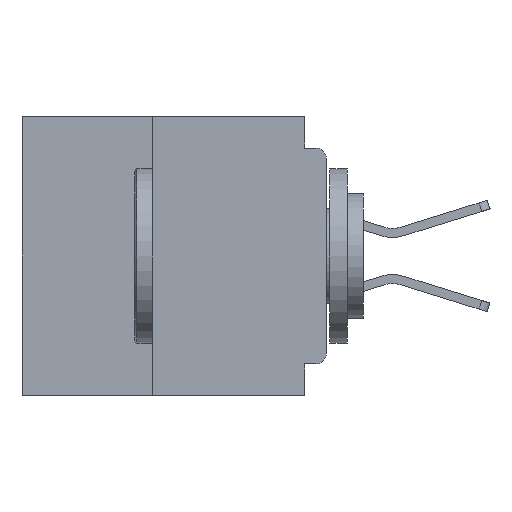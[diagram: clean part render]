
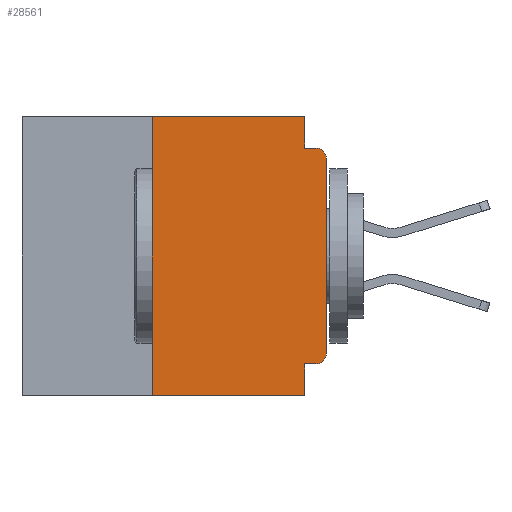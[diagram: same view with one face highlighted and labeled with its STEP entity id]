
A CAD part, left-side view. The second image highlights one B-rep face of the part: STEP entity #28561.
In plain terms, the highlighted planar face has unit normal (-1, 0, 0).
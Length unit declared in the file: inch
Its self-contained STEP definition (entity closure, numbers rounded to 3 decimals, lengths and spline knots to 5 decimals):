
#511 = ORIENTED_EDGE ( 'NONE', *, *, #9214, .T. ) ;
#1726 = VERTEX_POINT ( 'NONE', #33246 ) ;
#2229 = CARTESIAN_POINT ( 'NONE',  ( 0., 0.015, -0.34 ) ) ;
#2244 = DIRECTION ( 'NONE',  ( 0., 0., -1. ) ) ;
#4457 = VERTEX_POINT ( 'NONE', #42054 ) ;
#4629 = LINE ( 'NONE', #41701, #37160 ) ;
#4651 = CIRCLE ( 'NONE', #56440, 0.015 ) ;
#6211 = ORIENTED_EDGE ( 'NONE', *, *, #53278, .T. ) ;
#6963 = DIRECTION ( 'NONE',  ( 0., 0., -1. ) ) ;
#7548 = VERTEX_POINT ( 'NONE', #15556 ) ;
#9214 = EDGE_CURVE ( 'NONE', #54362, #4457, #4651, .T. ) ;
#9783 = LINE ( 'NONE', #13662, #20650 ) ;
#11473 = CARTESIAN_POINT ( 'NONE',  ( 0., 0.437, 0. ) ) ;
#12252 = VERTEX_POINT ( 'NONE', #59589 ) ;
#13662 = CARTESIAN_POINT ( 'NONE',  ( 0., 0.031, -0.4 ) ) ;
#14391 = VERTEX_POINT ( 'NONE', #35220 ) ;
#15294 = EDGE_CURVE ( 'NONE', #30630, #55558, #15785, .T. ) ;
#15556 = CARTESIAN_POINT ( 'NONE',  ( 0., 0.031, -0.355 ) ) ;
#15703 = ORIENTED_EDGE ( 'NONE', *, *, #23581, .T. ) ;
#15785 = LINE ( 'NONE', #46834, #38811 ) ;
#18201 = CARTESIAN_POINT ( 'NONE',  ( 0., 0., -0.06 ) ) ;
#19279 = CARTESIAN_POINT ( 'NONE',  ( 0., 0., 0. ) ) ;
#20650 = VECTOR ( 'NONE', #50344, 39.37008 ) ;
#20731 = ORIENTED_EDGE ( 'NONE', *, *, #15294, .F. ) ;
#21067 = VECTOR ( 'NONE', #23944, 39.37008 ) ;
#21116 = ORIENTED_EDGE ( 'NONE', *, *, #21518, .F. ) ;
#21518 = EDGE_CURVE ( 'NONE', #50332, #12252, #4629, .T. ) ;
#21845 = DIRECTION ( 'NONE',  ( 0., -1., 0. ) ) ;
#22014 = VECTOR ( 'NONE', #54327, 39.37008 ) ;
#22151 = EDGE_LOOP ( 'NONE', ( #15703, #511, #33731, #21116, #30706, #20731, #6211, #42211, #29672, #48506 ) ) ;
#22494 = LINE ( 'NONE', #29238, #30462 ) ;
#22687 = LINE ( 'NONE', #53806, #44177 ) ;
#23581 = EDGE_CURVE ( 'NONE', #14391, #54362, #57522, .T. ) ;
#23944 = DIRECTION ( 'NONE',  ( 0., 0., 1. ) ) ;
#24958 = AXIS2_PLACEMENT_3D ( 'NONE', #2229, #34638, #6963 ) ;
#25932 = DIRECTION ( 'NONE',  ( -1., 0., 0. ) ) ;
#27674 = CARTESIAN_POINT ( 'NONE',  ( 0., 0.25, 0. ) ) ;
#28421 = CARTESIAN_POINT ( 'NONE',  ( 0., 0.031, 0. ) ) ;
#28561 = ADVANCED_FACE ( 'NONE', ( #31415 ), #43609, .F. ) ;
#29238 = CARTESIAN_POINT ( 'NONE',  ( 0., 0.437, -0.4 ) ) ;
#29376 = CARTESIAN_POINT ( 'NONE',  ( 0., 0.25, -0.4 ) ) ;
#29672 = ORIENTED_EDGE ( 'NONE', *, *, #33974, .F. ) ;
#30059 = DIRECTION ( 'NONE',  ( 1., 0., 0. ) ) ;
#30462 = VECTOR ( 'NONE', #38232, 39.37008 ) ;
#30630 = VERTEX_POINT ( 'NONE', #29376 ) ;
#30706 = ORIENTED_EDGE ( 'NONE', *, *, #41663, .F. ) ;
#31415 = FACE_OUTER_BOUND ( 'NONE', #22151, .T. ) ;
#33246 = CARTESIAN_POINT ( 'NONE',  ( 0., 0.015, -0.355 ) ) ;
#33731 = ORIENTED_EDGE ( 'NONE', *, *, #58367, .F. ) ;
#33974 = EDGE_CURVE ( 'NONE', #1726, #7548, #46359, .T. ) ;
#34151 = DIRECTION ( 'NONE',  ( 0., -1., 0. ) ) ;
#34638 = DIRECTION ( 'NONE',  ( -1., 0., 0. ) ) ;
#35149 = VECTOR ( 'NONE', #34151, 39.37008 ) ;
#35220 = CARTESIAN_POINT ( 'NONE',  ( 0., 0., -0.34 ) ) ;
#37160 = VECTOR ( 'NONE', #46275, 39.37008 ) ;
#38232 = DIRECTION ( 'NONE',  ( 0., -1., 0. ) ) ;
#38273 = CARTESIAN_POINT ( 'NONE',  ( 0., 0.031, -0.4 ) ) ;
#38811 = VECTOR ( 'NONE', #51406, 39.37008 ) ;
#39716 = CIRCLE ( 'NONE', #24958, 0.015 ) ;
#41663 = EDGE_CURVE ( 'NONE', #55558, #50332, #22687, .T. ) ;
#41701 = CARTESIAN_POINT ( 'NONE',  ( 0., 0.031, 0. ) ) ;
#42054 = CARTESIAN_POINT ( 'NONE',  ( 0., 0.015, -0.045 ) ) ;
#42211 = ORIENTED_EDGE ( 'NONE', *, *, #50234, .F. ) ;
#43609 = PLANE ( 'NONE',  #55930 ) ;
#44177 = VECTOR ( 'NONE', #21845, 39.37008 ) ;
#46275 = DIRECTION ( 'NONE',  ( 0., 0., -1. ) ) ;
#46359 = LINE ( 'NONE', #49767, #22014 ) ;
#46834 = CARTESIAN_POINT ( 'NONE',  ( 0., 0.25, -0.4 ) ) ;
#47224 = LINE ( 'NONE', #47659, #35149 ) ;
#47659 = CARTESIAN_POINT ( 'NONE',  ( 0., 0., -0.045 ) ) ;
#48506 = ORIENTED_EDGE ( 'NONE', *, *, #53385, .T. ) ;
#49767 = CARTESIAN_POINT ( 'NONE',  ( 0., 0., -0.355 ) ) ;
#49843 = VERTEX_POINT ( 'NONE', #38273 ) ;
#50234 = EDGE_CURVE ( 'NONE', #7548, #49843, #9783, .T. ) ;
#50332 = VERTEX_POINT ( 'NONE', #28421 ) ;
#50344 = DIRECTION ( 'NONE',  ( 0., 0., -1. ) ) ;
#51406 = DIRECTION ( 'NONE',  ( 0., 0., 1. ) ) ;
#53244 = CARTESIAN_POINT ( 'NONE',  ( 0., 0.015, -0.06 ) ) ;
#53278 = EDGE_CURVE ( 'NONE', #30630, #49843, #22494, .T. ) ;
#53385 = EDGE_CURVE ( 'NONE', #1726, #14391, #39716, .T. ) ;
#53806 = CARTESIAN_POINT ( 'NONE',  ( 0., 0.437, 0. ) ) ;
#54327 = DIRECTION ( 'NONE',  ( 0., 1., 0. ) ) ;
#54362 = VERTEX_POINT ( 'NONE', #18201 ) ;
#55558 = VERTEX_POINT ( 'NONE', #27674 ) ;
#55930 = AXIS2_PLACEMENT_3D ( 'NONE', #11473, #30059, #2244 ) ;
#56440 = AXIS2_PLACEMENT_3D ( 'NONE', #53244, #25932, #57835 ) ;
#57522 = LINE ( 'NONE', #19279, #21067 ) ;
#57835 = DIRECTION ( 'NONE',  ( 0., 0., -1. ) ) ;
#58367 = EDGE_CURVE ( 'NONE', #12252, #4457, #47224, .T. ) ;
#59589 = CARTESIAN_POINT ( 'NONE',  ( 0., 0.031, -0.045 ) ) ;
